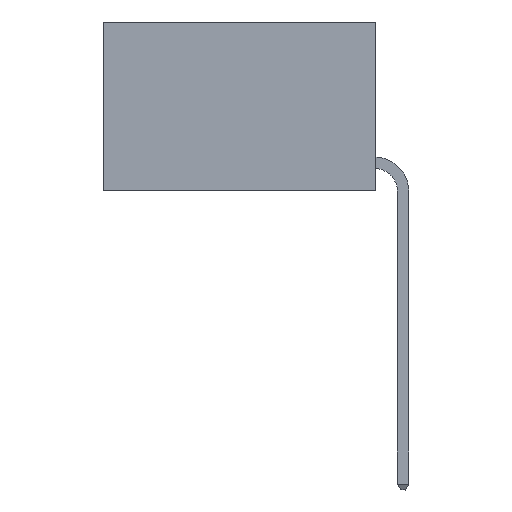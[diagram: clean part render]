
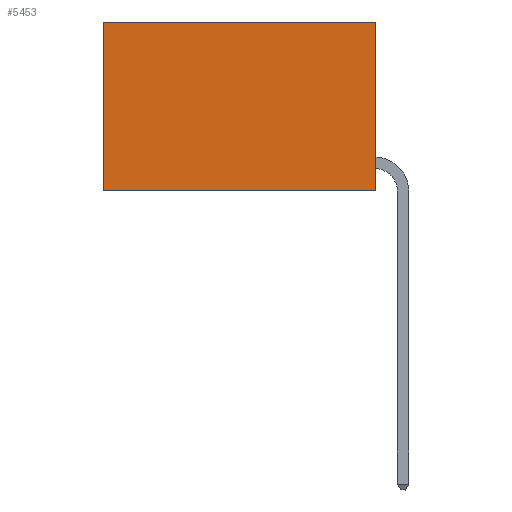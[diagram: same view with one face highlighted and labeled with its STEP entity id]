
A CAD part, left-side view. The second image highlights one B-rep face of the part: STEP entity #5453.
In plain terms, the highlighted planar face has unit normal (-1, 0, 0).
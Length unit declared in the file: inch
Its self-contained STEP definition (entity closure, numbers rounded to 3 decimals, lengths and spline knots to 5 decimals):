
#76 = VECTOR ( 'NONE', #17867, 39.37008 ) ;
#642 = CARTESIAN_POINT ( 'NONE',  ( 0.2625, 0., 0. ) ) ;
#998 = VERTEX_POINT ( 'NONE', #8942 ) ;
#2711 = CARTESIAN_POINT ( 'NONE',  ( 0.2625, 0.6, 0. ) ) ;
#4851 = EDGE_CURVE ( 'NONE', #998, #8600, #25638, .T. ) ;
#4956 = DIRECTION ( 'NONE',  ( 0., 0., -1. ) ) ;
#5453 = ADVANCED_FACE ( 'NONE', ( #26579 ), #20932, .F. ) ;
#6723 = LINE ( 'NONE', #642, #23369 ) ;
#7192 = CARTESIAN_POINT ( 'NONE',  ( 0.2625, 0., -0.37 ) ) ;
#8341 = LINE ( 'NONE', #2711, #19327 ) ;
#8600 = VERTEX_POINT ( 'NONE', #10194 ) ;
#8942 = CARTESIAN_POINT ( 'NONE',  ( 0.2625, 0., 0. ) ) ;
#9959 = DIRECTION ( 'NONE',  ( 0., 0., -1. ) ) ;
#10194 = CARTESIAN_POINT ( 'NONE',  ( 0.2625, 0.6, 0. ) ) ;
#13151 = EDGE_CURVE ( 'NONE', #20528, #19795, #17102, .T. ) ;
#14434 = DIRECTION ( 'NONE',  ( 0., 1., 0. ) ) ;
#14638 = EDGE_CURVE ( 'NONE', #998, #20528, #6723, .T. ) ;
#14941 = ORIENTED_EDGE ( 'NONE', *, *, #22017, .T. ) ;
#15053 = ORIENTED_EDGE ( 'NONE', *, *, #13151, .F. ) ;
#15555 = ORIENTED_EDGE ( 'NONE', *, *, #14638, .F. ) ;
#15669 = ORIENTED_EDGE ( 'NONE', *, *, #4851, .T. ) ;
#17102 = LINE ( 'NONE', #25959, #76 ) ;
#17112 = AXIS2_PLACEMENT_3D ( 'NONE', #27209, #23049, #9959 ) ;
#17550 = CARTESIAN_POINT ( 'NONE',  ( 0.2625, 0.6, -0.37 ) ) ;
#17867 = DIRECTION ( 'NONE',  ( 0., 1., 0. ) ) ;
#18247 = DIRECTION ( 'NONE',  ( 0., 0., -1. ) ) ;
#19327 = VECTOR ( 'NONE', #4956, 39.37008 ) ;
#19795 = VERTEX_POINT ( 'NONE', #17550 ) ;
#20528 = VERTEX_POINT ( 'NONE', #7192 ) ;
#20932 = PLANE ( 'NONE',  #17112 ) ;
#20969 = CARTESIAN_POINT ( 'NONE',  ( 0.2625, 0., 0. ) ) ;
#22017 = EDGE_CURVE ( 'NONE', #8600, #19795, #8341, .T. ) ;
#23049 = DIRECTION ( 'NONE',  ( 1., 0., 0. ) ) ;
#23369 = VECTOR ( 'NONE', #18247, 39.37008 ) ;
#24937 = VECTOR ( 'NONE', #14434, 39.37008 ) ;
#25399 = EDGE_LOOP ( 'NONE', ( #14941, #15053, #15555, #15669 ) ) ;
#25638 = LINE ( 'NONE', #20969, #24937 ) ;
#25959 = CARTESIAN_POINT ( 'NONE',  ( 0.2625, 0., -0.37 ) ) ;
#26579 = FACE_OUTER_BOUND ( 'NONE', #25399, .T. ) ;
#27209 = CARTESIAN_POINT ( 'NONE',  ( 0.2625, 0., 0. ) ) ;
